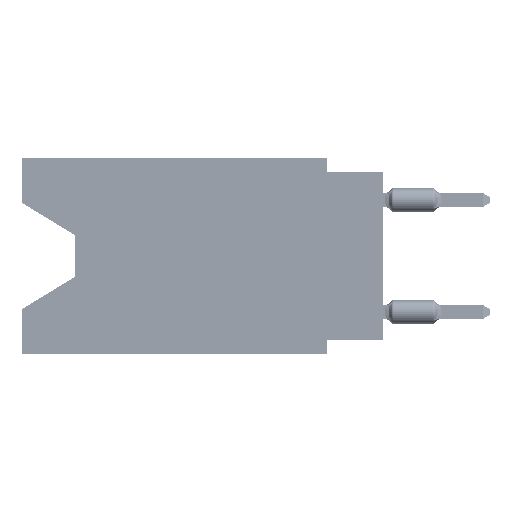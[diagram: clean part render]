
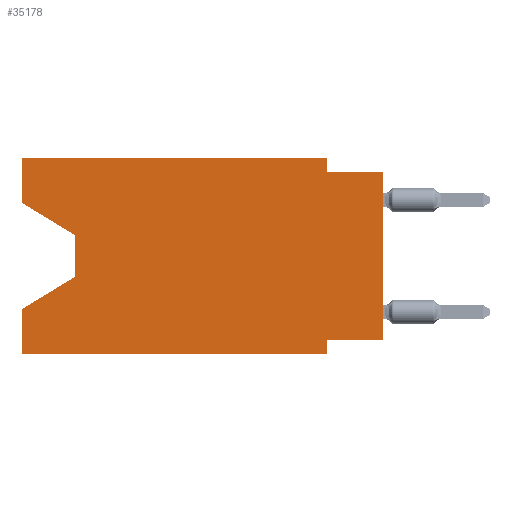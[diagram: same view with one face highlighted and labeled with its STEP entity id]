
A CAD part, left-side view. The second image highlights one B-rep face of the part: STEP entity #35178.
In plain terms, the highlighted planar face has unit normal (-1, 0, 0).
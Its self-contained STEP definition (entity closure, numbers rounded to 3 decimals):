
#2708 = DIRECTION ( 'NONE',  ( 0., 0., 1. ) ) ;
#3270 = LINE ( 'NONE', #29475, #11278 ) ;
#3760 = CARTESIAN_POINT ( 'NONE',  ( 0., 16.383, 0. ) ) ;
#4391 = EDGE_CURVE ( 'NONE', #39162, #26720, #68570, .T. ) ;
#9344 = ORIENTED_EDGE ( 'NONE', *, *, #51742, .T. ) ;
#10113 = LINE ( 'NONE', #63314, #80612 ) ;
#10585 = PLANE ( 'NONE',  #37022 ) ;
#11278 = VECTOR ( 'NONE', #42107, 1000. ) ;
#11289 = VERTEX_POINT ( 'NONE', #16784 ) ;
#11495 = VECTOR ( 'NONE', #19667, 1000. ) ;
#12140 = VECTOR ( 'NONE', #76106, 1000. ) ;
#15531 = VECTOR ( 'NONE', #86165, 1000. ) ;
#15945 = CARTESIAN_POINT ( 'NONE',  ( 0., 0., -8.255 ) ) ;
#16274 = DIRECTION ( 'NONE',  ( 0., 0., -1. ) ) ;
#16468 = DIRECTION ( 'NONE',  ( 0., 0., -1. ) ) ;
#16479 = CARTESIAN_POINT ( 'NONE',  ( 0., 16.383, -2.038 ) ) ;
#16784 = CARTESIAN_POINT ( 'NONE',  ( 0., 13.97, -3.505 ) ) ;
#18641 = EDGE_LOOP ( 'NONE', ( #51164, #36971, #9344, #73776, #57271, #82126, #30542, #31264, #75908, #61537, #77531, #51443 ) ) ;
#19667 = DIRECTION ( 'NONE',  ( 0., 0., 1. ) ) ;
#19746 = VERTEX_POINT ( 'NONE', #54613 ) ;
#21978 = VERTEX_POINT ( 'NONE', #74669 ) ;
#22388 = CARTESIAN_POINT ( 'NONE',  ( 0., 16.383, 0. ) ) ;
#23035 = EDGE_CURVE ( 'NONE', #19746, #55987, #45214, .T. ) ;
#23898 = VERTEX_POINT ( 'NONE', #79738 ) ;
#24337 = VECTOR ( 'NONE', #74255, 1000. ) ;
#26417 = VECTOR ( 'NONE', #36523, 1000. ) ;
#26720 = VERTEX_POINT ( 'NONE', #72950 ) ;
#29475 = CARTESIAN_POINT ( 'NONE',  ( 0., 13.97, -3.505 ) ) ;
#29840 = VERTEX_POINT ( 'NONE', #61330 ) ;
#29950 = LINE ( 'NONE', #3760, #62581 ) ;
#30226 = CARTESIAN_POINT ( 'NONE',  ( 0., 16.383, -8.89 ) ) ;
#30260 = LINE ( 'NONE', #49867, #46523 ) ;
#30542 = ORIENTED_EDGE ( 'NONE', *, *, #38588, .F. ) ;
#31264 = ORIENTED_EDGE ( 'NONE', *, *, #64727, .T. ) ;
#32994 = EDGE_CURVE ( 'NONE', #74251, #37756, #41975, .T. ) ;
#35178 = ADVANCED_FACE ( 'NONE', ( #70756 ), #10585, .F. ) ;
#35443 = CARTESIAN_POINT ( 'NONE',  ( 0., 16.383, -8.89 ) ) ;
#35883 = CARTESIAN_POINT ( 'NONE',  ( 0., 16.383, 0. ) ) ;
#36523 = DIRECTION ( 'NONE',  ( 0., -0.855, -0.519 ) ) ;
#36606 = CARTESIAN_POINT ( 'NONE',  ( 0., 16.383, -2.038 ) ) ;
#36971 = ORIENTED_EDGE ( 'NONE', *, *, #43871, .T. ) ;
#37022 = AXIS2_PLACEMENT_3D ( 'NONE', #62469, #49832, #16274 ) ;
#37756 = VERTEX_POINT ( 'NONE', #22388 ) ;
#38588 = EDGE_CURVE ( 'NONE', #21978, #42005, #80600, .T. ) ;
#38822 = CARTESIAN_POINT ( 'NONE',  ( 0., 13.97, -5.385 ) ) ;
#39162 = VERTEX_POINT ( 'NONE', #30226 ) ;
#39517 = VECTOR ( 'NONE', #2708, 1000. ) ;
#41423 = EDGE_CURVE ( 'NONE', #29840, #19746, #10113, .T. ) ;
#41975 = LINE ( 'NONE', #35883, #39517 ) ;
#42005 = VERTEX_POINT ( 'NONE', #44878 ) ;
#42065 = CARTESIAN_POINT ( 'NONE',  ( 0., 16.383, -6.852 ) ) ;
#42107 = DIRECTION ( 'NONE',  ( 0., 0., -1. ) ) ;
#42256 = EDGE_CURVE ( 'NONE', #74251, #11289, #62243, .T. ) ;
#43871 = EDGE_CURVE ( 'NONE', #11289, #23898, #3270, .T. ) ;
#44305 = DIRECTION ( 'NONE',  ( 0., 0., 1. ) ) ;
#44878 = CARTESIAN_POINT ( 'NONE',  ( 0., 2.54, -8.255 ) ) ;
#45214 = LINE ( 'NONE', #59152, #15531 ) ;
#46523 = VECTOR ( 'NONE', #62509, 1000. ) ;
#46661 = VECTOR ( 'NONE', #64986, 1000. ) ;
#49832 = DIRECTION ( 'NONE',  ( 1., 0., 0. ) ) ;
#49867 = CARTESIAN_POINT ( 'NONE',  ( 0., 16.383, 0. ) ) ;
#51164 = ORIENTED_EDGE ( 'NONE', *, *, #42256, .T. ) ;
#51443 = ORIENTED_EDGE ( 'NONE', *, *, #32994, .F. ) ;
#51742 = EDGE_CURVE ( 'NONE', #23898, #63179, #73233, .T. ) ;
#52816 = EDGE_CURVE ( 'NONE', #37756, #29840, #30260, .T. ) ;
#54613 = CARTESIAN_POINT ( 'NONE',  ( 0., 2.54, -0.635 ) ) ;
#55987 = VERTEX_POINT ( 'NONE', #79152 ) ;
#57271 = ORIENTED_EDGE ( 'NONE', *, *, #4391, .T. ) ;
#59152 = CARTESIAN_POINT ( 'NONE',  ( 0., 0., -0.635 ) ) ;
#59339 = CARTESIAN_POINT ( 'NONE',  ( 0., 0., 0. ) ) ;
#61330 = CARTESIAN_POINT ( 'NONE',  ( 0., 2.54, 0. ) ) ;
#61361 = CARTESIAN_POINT ( 'NONE',  ( 0., 2.54, -8.89 ) ) ;
#61537 = ORIENTED_EDGE ( 'NONE', *, *, #41423, .F. ) ;
#62243 = LINE ( 'NONE', #16479, #26417 ) ;
#62469 = CARTESIAN_POINT ( 'NONE',  ( 0., 16.383, 0. ) ) ;
#62509 = DIRECTION ( 'NONE',  ( 0., -1., 0. ) ) ;
#62581 = VECTOR ( 'NONE', #44305, 1000. ) ;
#63179 = VERTEX_POINT ( 'NONE', #42065 ) ;
#63314 = CARTESIAN_POINT ( 'NONE',  ( 0., 2.54, 0. ) ) ;
#64727 = EDGE_CURVE ( 'NONE', #21978, #55987, #72434, .T. ) ;
#64986 = DIRECTION ( 'NONE',  ( 0., 0.855, -0.519 ) ) ;
#66989 = VECTOR ( 'NONE', #16468, 1000. ) ;
#68570 = LINE ( 'NONE', #35443, #24337 ) ;
#70290 = DIRECTION ( 'NONE',  ( 0., 0., -1. ) ) ;
#70756 = FACE_OUTER_BOUND ( 'NONE', #18641, .T. ) ;
#72434 = LINE ( 'NONE', #59339, #11495 ) ;
#72950 = CARTESIAN_POINT ( 'NONE',  ( 0., 2.54, -8.89 ) ) ;
#73233 = LINE ( 'NONE', #38822, #46661 ) ;
#73776 = ORIENTED_EDGE ( 'NONE', *, *, #77800, .F. ) ;
#74251 = VERTEX_POINT ( 'NONE', #36606 ) ;
#74255 = DIRECTION ( 'NONE',  ( 0., -1., 0. ) ) ;
#74669 = CARTESIAN_POINT ( 'NONE',  ( 0., 0., -8.255 ) ) ;
#75908 = ORIENTED_EDGE ( 'NONE', *, *, #23035, .F. ) ;
#76106 = DIRECTION ( 'NONE',  ( 0., 1., 0. ) ) ;
#76186 = LINE ( 'NONE', #61361, #66989 ) ;
#77531 = ORIENTED_EDGE ( 'NONE', *, *, #52816, .F. ) ;
#77800 = EDGE_CURVE ( 'NONE', #39162, #63179, #29950, .T. ) ;
#79152 = CARTESIAN_POINT ( 'NONE',  ( 0., 0., -0.635 ) ) ;
#79738 = CARTESIAN_POINT ( 'NONE',  ( 0., 13.97, -5.385 ) ) ;
#80079 = EDGE_CURVE ( 'NONE', #42005, #26720, #76186, .T. ) ;
#80600 = LINE ( 'NONE', #15945, #12140 ) ;
#80612 = VECTOR ( 'NONE', #70290, 1000. ) ;
#82126 = ORIENTED_EDGE ( 'NONE', *, *, #80079, .F. ) ;
#86165 = DIRECTION ( 'NONE',  ( 0., -1., 0. ) ) ;
